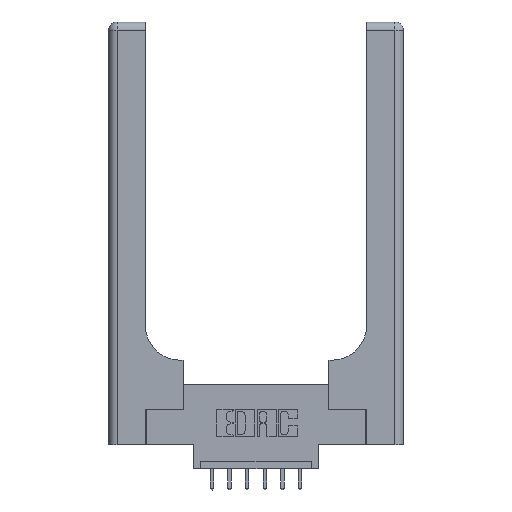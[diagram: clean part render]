
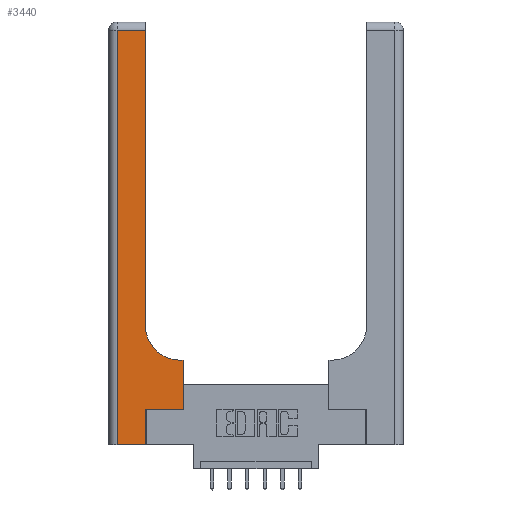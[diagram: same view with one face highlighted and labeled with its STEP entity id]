
A CAD part, top view. The second image highlights one B-rep face of the part: STEP entity #3440.
In plain terms, the highlighted planar face has unit normal (0, 0, 1).
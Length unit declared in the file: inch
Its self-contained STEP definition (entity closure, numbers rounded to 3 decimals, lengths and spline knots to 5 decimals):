
#127 = ORIENTED_EDGE ( 'NONE', *, *, #1571, .T. ) ;
#167 = PLANE ( 'NONE',  #3298 ) ;
#190 = DIRECTION ( 'NONE',  ( 1., 0., 0. ) ) ;
#437 = CARTESIAN_POINT ( 'NONE',  ( 0.265, 0., 0.37 ) ) ;
#489 = CARTESIAN_POINT ( 'NONE',  ( 0.265, 0.25, 0.37 ) ) ;
#631 = DIRECTION ( 'NONE',  ( 1., 0., 0. ) ) ;
#657 = VERTEX_POINT ( 'NONE', #11041 ) ;
#696 = VECTOR ( 'NONE', #10266, 39.37008 ) ;
#760 = VERTEX_POINT ( 'NONE', #12500 ) ;
#813 = VECTOR ( 'NONE', #1531, 39.37008 ) ;
#862 = CARTESIAN_POINT ( 'NONE',  ( 0., 2.94, 0.37 ) ) ;
#1531 = DIRECTION ( 'NONE',  ( 0., 1., 0. ) ) ;
#1571 = EDGE_CURVE ( 'NONE', #9298, #760, #10405, .T. ) ;
#1620 = ORIENTED_EDGE ( 'NONE', *, *, #11073, .T. ) ;
#2241 = CARTESIAN_POINT ( 'NONE',  ( 0., 0., 0.37 ) ) ;
#2394 = ORIENTED_EDGE ( 'NONE', *, *, #3978, .T. ) ;
#2630 = CARTESIAN_POINT ( 'NONE',  ( 0.26, 0.6, 0.37 ) ) ;
#3063 = VERTEX_POINT ( 'NONE', #3085 ) ;
#3085 = CARTESIAN_POINT ( 'NONE',  ( 0.528, 0.6, 0.37 ) ) ;
#3298 = AXIS2_PLACEMENT_3D ( 'NONE', #13445, #7919, #10168 ) ;
#3440 = ADVANCED_FACE ( 'NONE', ( #6679 ), #167, .F. ) ;
#3489 = VERTEX_POINT ( 'NONE', #9945 ) ;
#3781 = VECTOR ( 'NONE', #12205, 39.37008 ) ;
#3978 = EDGE_CURVE ( 'NONE', #14347, #9298, #11391, .T. ) ;
#4214 = AXIS2_PLACEMENT_3D ( 'NONE', #6122, #10549, #631 ) ;
#4372 = VECTOR ( 'NONE', #7441, 39.37008 ) ;
#4740 = CARTESIAN_POINT ( 'NONE',  ( 0.26, 3., 0.37 ) ) ;
#5256 = LINE ( 'NONE', #14189, #10086 ) ;
#5265 = LINE ( 'NONE', #9699, #10082 ) ;
#6122 = CARTESIAN_POINT ( 'NONE',  ( 0.51, 0.85, 0.37 ) ) ;
#6288 = ORIENTED_EDGE ( 'NONE', *, *, #11134, .T. ) ;
#6303 = CARTESIAN_POINT ( 'NONE',  ( 0.06, 2.94, 0.37 ) ) ;
#6503 = EDGE_LOOP ( 'NONE', ( #127, #7193, #10849, #13612, #1620, #6612, #6288, #11016, #2394 ) ) ;
#6612 = ORIENTED_EDGE ( 'NONE', *, *, #13861, .T. ) ;
#6679 = FACE_OUTER_BOUND ( 'NONE', #6503, .T. ) ;
#7112 = DIRECTION ( 'NONE',  ( -1., 0., 0. ) ) ;
#7193 = ORIENTED_EDGE ( 'NONE', *, *, #7276, .T. ) ;
#7276 = EDGE_CURVE ( 'NONE', #760, #11957, #8700, .T. ) ;
#7441 = DIRECTION ( 'NONE',  ( -1., 0., 0. ) ) ;
#7919 = DIRECTION ( 'NONE',  ( 0., 0., -1. ) ) ;
#8700 = LINE ( 'NONE', #862, #4372 ) ;
#9077 = VERTEX_POINT ( 'NONE', #489 ) ;
#9298 = VERTEX_POINT ( 'NONE', #10987 ) ;
#9580 = LINE ( 'NONE', #14006, #3781 ) ;
#9691 = DIRECTION ( 'NONE',  ( 1., 0., 0. ) ) ;
#9699 = CARTESIAN_POINT ( 'NONE',  ( 0.528, 0.25, 0.37 ) ) ;
#9945 = CARTESIAN_POINT ( 'NONE',  ( 0.265, 0., 0.37 ) ) ;
#10082 = VECTOR ( 'NONE', #12918, 39.37008 ) ;
#10086 = VECTOR ( 'NONE', #9691, 39.37008 ) ;
#10168 = DIRECTION ( 'NONE',  ( -1., 0., 0. ) ) ;
#10265 = VERTEX_POINT ( 'NONE', #13467 ) ;
#10266 = DIRECTION ( 'NONE',  ( 0., 1., 0. ) ) ;
#10297 = EDGE_CURVE ( 'NONE', #657, #3489, #11280, .T. ) ;
#10405 = LINE ( 'NONE', #4740, #696 ) ;
#10549 = DIRECTION ( 'NONE',  ( 0., 0., -1. ) ) ;
#10725 = EDGE_CURVE ( 'NONE', #3063, #14347, #12507, .T. ) ;
#10849 = ORIENTED_EDGE ( 'NONE', *, *, #12969, .T. ) ;
#10987 = CARTESIAN_POINT ( 'NONE',  ( 0.26, 0.85, 0.37 ) ) ;
#11016 = ORIENTED_EDGE ( 'NONE', *, *, #10725, .T. ) ;
#11041 = CARTESIAN_POINT ( 'NONE',  ( 0.06, 0., 0.37 ) ) ;
#11073 = EDGE_CURVE ( 'NONE', #3489, #9077, #11441, .T. ) ;
#11134 = EDGE_CURVE ( 'NONE', #10265, #3063, #5265, .T. ) ;
#11280 = LINE ( 'NONE', #2241, #12162 ) ;
#11391 = CIRCLE ( 'NONE', #4214, 0.25 ) ;
#11441 = LINE ( 'NONE', #437, #813 ) ;
#11957 = VERTEX_POINT ( 'NONE', #6303 ) ;
#12162 = VECTOR ( 'NONE', #190, 39.37008 ) ;
#12205 = DIRECTION ( 'NONE',  ( 0., -1., 0. ) ) ;
#12409 = VECTOR ( 'NONE', #7112, 39.37008 ) ;
#12500 = CARTESIAN_POINT ( 'NONE',  ( 0.26, 2.94, 0.37 ) ) ;
#12507 = LINE ( 'NONE', #2630, #12409 ) ;
#12918 = DIRECTION ( 'NONE',  ( 0., 1., 0. ) ) ;
#12969 = EDGE_CURVE ( 'NONE', #11957, #657, #9580, .T. ) ;
#13445 = CARTESIAN_POINT ( 'NONE',  ( 0., 3., 0.37 ) ) ;
#13467 = CARTESIAN_POINT ( 'NONE',  ( 0.528, 0.25, 0.37 ) ) ;
#13612 = ORIENTED_EDGE ( 'NONE', *, *, #10297, .T. ) ;
#13861 = EDGE_CURVE ( 'NONE', #9077, #10265, #5256, .T. ) ;
#14006 = CARTESIAN_POINT ( 'NONE',  ( 0.06, 3., 0.37 ) ) ;
#14189 = CARTESIAN_POINT ( 'NONE',  ( 0.265, 0.25, 0.37 ) ) ;
#14312 = CARTESIAN_POINT ( 'NONE',  ( 0.51, 0.6, 0.37 ) ) ;
#14347 = VERTEX_POINT ( 'NONE', #14312 ) ;
